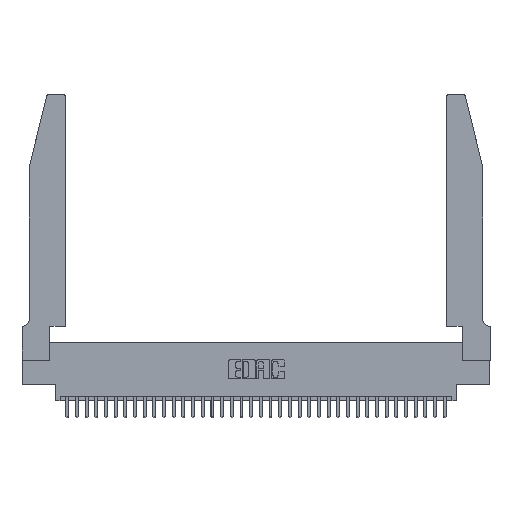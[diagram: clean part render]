
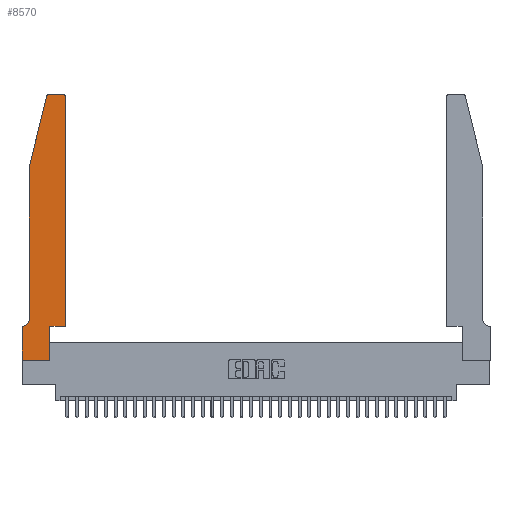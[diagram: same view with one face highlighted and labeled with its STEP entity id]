
A CAD part, top view. The second image highlights one B-rep face of the part: STEP entity #8570.
In plain terms, the highlighted planar face has unit normal (0, 0, 1).
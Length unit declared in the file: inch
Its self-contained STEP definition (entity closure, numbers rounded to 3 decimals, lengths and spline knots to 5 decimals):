
#175 = VERTEX_POINT ( 'NONE', #36288 ) ;
#689 = VECTOR ( 'NONE', #9265, 39.37008 ) ;
#930 = CARTESIAN_POINT ( 'NONE',  ( 0.4505, 2.72, 0.37 ) ) ;
#1173 = VERTEX_POINT ( 'NONE', #24420 ) ;
#1469 = VECTOR ( 'NONE', #7182, 39.37008 ) ;
#1776 = CARTESIAN_POINT ( 'NONE',  ( 0., 0.35, 0.37 ) ) ;
#2548 = ORIENTED_EDGE ( 'NONE', *, *, #10917, .T. ) ;
#2718 = ORIENTED_EDGE ( 'NONE', *, *, #35022, .T. ) ;
#2882 = CIRCLE ( 'NONE', #19985, 0.03 ) ;
#3149 = EDGE_LOOP ( 'NONE', ( #9298, #2548, #23142, #2718, #10533, #30184, #10260, #6726, #15142, #13686, #36100, #24869 ) ) ;
#3409 = VECTOR ( 'NONE', #9572, 39.37008 ) ;
#3516 = CARTESIAN_POINT ( 'NONE',  ( 0.0755, 2., 0.37 ) ) ;
#4119 = EDGE_CURVE ( 'NONE', #24980, #35960, #33942, .T. ) ;
#4430 = DIRECTION ( 'NONE',  ( 1., 0., 0. ) ) ;
#4537 = VERTEX_POINT ( 'NONE', #930 ) ;
#4618 = CARTESIAN_POINT ( 'NONE',  ( 0.2865, 0.35, 0.37 ) ) ;
#4803 = VERTEX_POINT ( 'NONE', #3516 ) ;
#4958 = CARTESIAN_POINT ( 'NONE',  ( 0.4505, 0.35, 0.37 ) ) ;
#6443 = AXIS2_PLACEMENT_3D ( 'NONE', #1776, #32497, #26941 ) ;
#6726 = ORIENTED_EDGE ( 'NONE', *, *, #28465, .T. ) ;
#7048 = EDGE_CURVE ( 'NONE', #1173, #24437, #35495, .T. ) ;
#7182 = DIRECTION ( 'NONE',  ( 0., 1., 0. ) ) ;
#7529 = VERTEX_POINT ( 'NONE', #12119 ) ;
#7757 = CIRCLE ( 'NONE', #33147, 0.03 ) ;
#8472 = VERTEX_POINT ( 'NONE', #11049 ) ;
#8570 = ADVANCED_FACE ( 'NONE', ( #11069 ), #23577, .T. ) ;
#8575 = DIRECTION ( 'NONE',  ( 1., 0., 0. ) ) ;
#9065 = EDGE_CURVE ( 'NONE', #8472, #175, #18469, .T. ) ;
#9265 = DIRECTION ( 'NONE',  ( 0., 1., 0. ) ) ;
#9298 = ORIENTED_EDGE ( 'NONE', *, *, #9065, .T. ) ;
#9572 = DIRECTION ( 'NONE',  ( -1., 0., 0. ) ) ;
#9788 = CARTESIAN_POINT ( 'NONE',  ( 0.4205, 2.72, 0.37 ) ) ;
#10260 = ORIENTED_EDGE ( 'NONE', *, *, #32035, .T. ) ;
#10309 = DIRECTION ( 'NONE',  ( -1., 0., 0. ) ) ;
#10466 = VECTOR ( 'NONE', #28890, 39.37008 ) ;
#10533 = ORIENTED_EDGE ( 'NONE', *, *, #26909, .T. ) ;
#10917 = EDGE_CURVE ( 'NONE', #175, #23612, #7757, .T. ) ;
#11011 = CARTESIAN_POINT ( 'NONE',  ( 0.0755, 0.35, 0.37 ) ) ;
#11049 = CARTESIAN_POINT ( 'NONE',  ( 0.4205, 2.75, 0.37 ) ) ;
#11069 = FACE_OUTER_BOUND ( 'NONE', #3149, .T. ) ;
#12119 = CARTESIAN_POINT ( 'NONE',  ( 0.2865, 0., 0.37 ) ) ;
#12610 = DIRECTION ( 'NONE',  ( 1., 0., 0. ) ) ;
#12689 = DIRECTION ( 'NONE',  ( 0., 0., 1. ) ) ;
#12896 = VECTOR ( 'NONE', #33545, 39.37008 ) ;
#13136 = CARTESIAN_POINT ( 'NONE',  ( 0.0055, 0.42, 0.37 ) ) ;
#13686 = ORIENTED_EDGE ( 'NONE', *, *, #4119, .T. ) ;
#14277 = CARTESIAN_POINT ( 'NONE',  ( 0., 0., 0.37 ) ) ;
#14946 = DIRECTION ( 'NONE',  ( 0., 0., 1. ) ) ;
#15122 = AXIS2_PLACEMENT_3D ( 'NONE', #13136, #21295, #10309 ) ;
#15142 = ORIENTED_EDGE ( 'NONE', *, *, #16679, .T. ) ;
#16402 = CARTESIAN_POINT ( 'NONE',  ( 0., 0., 0.37 ) ) ;
#16440 = CARTESIAN_POINT ( 'NONE',  ( 0.2605, 2.75, 0.37 ) ) ;
#16607 = LINE ( 'NONE', #35796, #1469 ) ;
#16679 = EDGE_CURVE ( 'NONE', #7529, #24980, #27872, .T. ) ;
#16690 = CARTESIAN_POINT ( 'NONE',  ( 0.25487, 2.72718, 0.37 ) ) ;
#16766 = DIRECTION ( 'NONE',  ( 1., 0., 0. ) ) ;
#16916 = CARTESIAN_POINT ( 'NONE',  ( 0.0755, 2., 0.37 ) ) ;
#17623 = LINE ( 'NONE', #16402, #18081 ) ;
#17716 = CIRCLE ( 'NONE', #15122, 0.07 ) ;
#18081 = VECTOR ( 'NONE', #16766, 39.37008 ) ;
#18310 = EDGE_CURVE ( 'NONE', #4537, #8472, #2882, .T. ) ;
#18466 = VECTOR ( 'NONE', #29294, 39.37008 ) ;
#18469 = LINE ( 'NONE', #16440, #3409 ) ;
#18790 = LINE ( 'NONE', #31092, #29402 ) ;
#19401 = LINE ( 'NONE', #29050, #18466 ) ;
#19739 = CARTESIAN_POINT ( 'NONE',  ( 0.0755, 0.42, 0.37 ) ) ;
#19985 = AXIS2_PLACEMENT_3D ( 'NONE', #9788, #14946, #12610 ) ;
#20031 = DIRECTION ( 'NONE',  ( 0., -1., 0. ) ) ;
#21295 = DIRECTION ( 'NONE',  ( 0., 0., -1. ) ) ;
#21463 = CARTESIAN_POINT ( 'NONE',  ( 0., 0.35, 0.37 ) ) ;
#23142 = ORIENTED_EDGE ( 'NONE', *, *, #30412, .T. ) ;
#23577 = PLANE ( 'NONE',  #6443 ) ;
#23612 = VERTEX_POINT ( 'NONE', #16690 ) ;
#23875 = CARTESIAN_POINT ( 'NONE',  ( 0.4505, 0.35, 0.37 ) ) ;
#24420 = CARTESIAN_POINT ( 'NONE',  ( 0.0055, 0.35, 0.37 ) ) ;
#24437 = VERTEX_POINT ( 'NONE', #21463 ) ;
#24869 = ORIENTED_EDGE ( 'NONE', *, *, #18310, .T. ) ;
#24980 = VERTEX_POINT ( 'NONE', #4618 ) ;
#26841 = CARTESIAN_POINT ( 'NONE',  ( 0.284, 2.72, 0.37 ) ) ;
#26851 = LINE ( 'NONE', #16916, #10466 ) ;
#26909 = EDGE_CURVE ( 'NONE', #28645, #1173, #17716, .T. ) ;
#26941 = DIRECTION ( 'NONE',  ( 1., 0., 0. ) ) ;
#27872 = LINE ( 'NONE', #31571, #689 ) ;
#28465 = EDGE_CURVE ( 'NONE', #31594, #7529, #17623, .T. ) ;
#28645 = VERTEX_POINT ( 'NONE', #19739 ) ;
#28890 = DIRECTION ( 'NONE',  ( 0., -1., 0. ) ) ;
#29050 = CARTESIAN_POINT ( 'NONE',  ( 0.0755, 2., 0.37 ) ) ;
#29294 = DIRECTION ( 'NONE',  ( -0.239, -0.971, 0. ) ) ;
#29402 = VECTOR ( 'NONE', #20031, 39.37008 ) ;
#30184 = ORIENTED_EDGE ( 'NONE', *, *, #7048, .T. ) ;
#30412 = EDGE_CURVE ( 'NONE', #23612, #4803, #19401, .T. ) ;
#31092 = CARTESIAN_POINT ( 'NONE',  ( 0., 0., 0.37 ) ) ;
#31571 = CARTESIAN_POINT ( 'NONE',  ( 0.2865, 0.35, 0.37 ) ) ;
#31594 = VERTEX_POINT ( 'NONE', #14277 ) ;
#31729 = EDGE_CURVE ( 'NONE', #35960, #4537, #16607, .T. ) ;
#32035 = EDGE_CURVE ( 'NONE', #24437, #31594, #18790, .T. ) ;
#32497 = DIRECTION ( 'NONE',  ( 0., 0., 1. ) ) ;
#33040 = VECTOR ( 'NONE', #8575, 39.37008 ) ;
#33147 = AXIS2_PLACEMENT_3D ( 'NONE', #26841, #12689, #4430 ) ;
#33545 = DIRECTION ( 'NONE',  ( -1., 0., 0. ) ) ;
#33942 = LINE ( 'NONE', #4958, #33040 ) ;
#35022 = EDGE_CURVE ( 'NONE', #4803, #28645, #26851, .T. ) ;
#35495 = LINE ( 'NONE', #11011, #12896 ) ;
#35796 = CARTESIAN_POINT ( 'NONE',  ( 0.4505, 0.35, 0.37 ) ) ;
#35960 = VERTEX_POINT ( 'NONE', #23875 ) ;
#36100 = ORIENTED_EDGE ( 'NONE', *, *, #31729, .T. ) ;
#36288 = CARTESIAN_POINT ( 'NONE',  ( 0.284, 2.75, 0.37 ) ) ;
